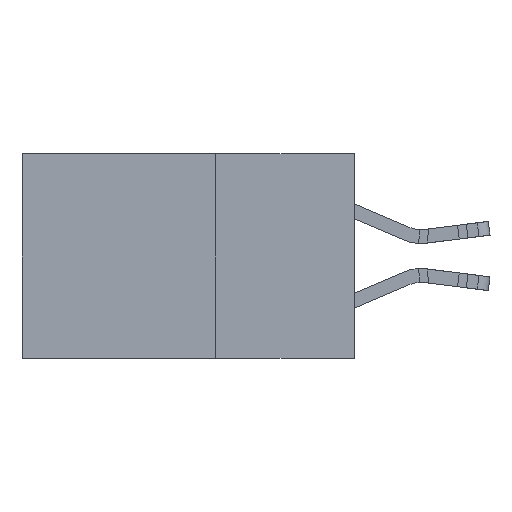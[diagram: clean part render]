
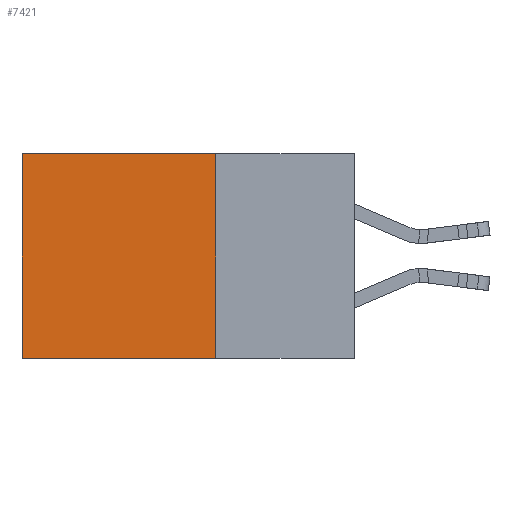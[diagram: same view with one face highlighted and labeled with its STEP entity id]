
A CAD part, left-side view. The second image highlights one B-rep face of the part: STEP entity #7421.
In plain terms, the highlighted planar face has unit normal (-1, 0, 0).
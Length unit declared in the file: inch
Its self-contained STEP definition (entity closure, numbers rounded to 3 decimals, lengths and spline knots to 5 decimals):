
#891 = DIRECTION ( 'NONE',  ( 1., 0., 0. ) ) ;
#2025 = FACE_OUTER_BOUND ( 'NONE', #7659, .T. ) ;
#2610 = EDGE_CURVE ( 'NONE', #17110, #6454, #10928, .T. ) ;
#2913 = PLANE ( 'NONE',  #11702 ) ;
#3332 = CARTESIAN_POINT ( 'NONE',  ( 0.2615, 0.6, -0.37 ) ) ;
#4284 = ORIENTED_EDGE ( 'NONE', *, *, #2610, .T. ) ;
#4503 = CARTESIAN_POINT ( 'NONE',  ( 0.2615, 0.6, -0.37 ) ) ;
#4768 = VECTOR ( 'NONE', #19470, 39.37008 ) ;
#5564 = DIRECTION ( 'NONE',  ( 0., 0., -1. ) ) ;
#6454 = VERTEX_POINT ( 'NONE', #4503 ) ;
#6969 = VECTOR ( 'NONE', #17487, 39.37008 ) ;
#7018 = LINE ( 'NONE', #20103, #10616 ) ;
#7421 = ADVANCED_FACE ( 'NONE', ( #2025 ), #2913, .F. ) ;
#7432 = EDGE_CURVE ( 'NONE', #21280, #6454, #7623, .T. ) ;
#7623 = LINE ( 'NONE', #15357, #6969 ) ;
#7659 = EDGE_LOOP ( 'NONE', ( #4284, #18412, #26618, #16121 ) ) ;
#8101 = DIRECTION ( 'NONE',  ( 0., 0., -1. ) ) ;
#9267 = CARTESIAN_POINT ( 'NONE',  ( 0.2615, 0.25, -0.37 ) ) ;
#10616 = VECTOR ( 'NONE', #5564, 39.37008 ) ;
#10928 = LINE ( 'NONE', #3332, #26680 ) ;
#11702 = AXIS2_PLACEMENT_3D ( 'NONE', #9267, #891, #15450 ) ;
#13300 = CARTESIAN_POINT ( 'NONE',  ( 0.2615, 0.25, 0. ) ) ;
#13774 = CARTESIAN_POINT ( 'NONE',  ( 0.2615, 0.25, 0. ) ) ;
#15357 = CARTESIAN_POINT ( 'NONE',  ( 0.2615, 0.25, -0.37 ) ) ;
#15450 = DIRECTION ( 'NONE',  ( 0., 0., -1. ) ) ;
#15709 = VERTEX_POINT ( 'NONE', #13774 ) ;
#16121 = ORIENTED_EDGE ( 'NONE', *, *, #20446, .T. ) ;
#16423 = EDGE_CURVE ( 'NONE', #15709, #21280, #7018, .T. ) ;
#17110 = VERTEX_POINT ( 'NONE', #24215 ) ;
#17487 = DIRECTION ( 'NONE',  ( 0., 1., 0. ) ) ;
#17619 = CARTESIAN_POINT ( 'NONE',  ( 0.2615, 0.25, -0.37 ) ) ;
#18412 = ORIENTED_EDGE ( 'NONE', *, *, #7432, .F. ) ;
#19470 = DIRECTION ( 'NONE',  ( 0., 1., 0. ) ) ;
#20103 = CARTESIAN_POINT ( 'NONE',  ( 0.2615, 0.25, -0.37 ) ) ;
#20446 = EDGE_CURVE ( 'NONE', #15709, #17110, #21278, .T. ) ;
#21278 = LINE ( 'NONE', #13300, #4768 ) ;
#21280 = VERTEX_POINT ( 'NONE', #17619 ) ;
#24215 = CARTESIAN_POINT ( 'NONE',  ( 0.2615, 0.6, 0. ) ) ;
#26618 = ORIENTED_EDGE ( 'NONE', *, *, #16423, .F. ) ;
#26680 = VECTOR ( 'NONE', #8101, 39.37008 ) ;
